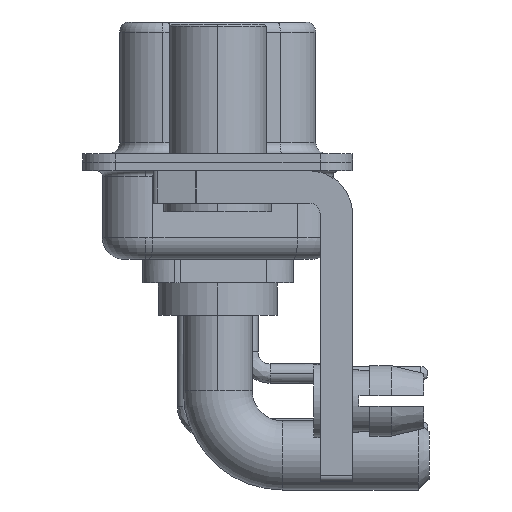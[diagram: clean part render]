
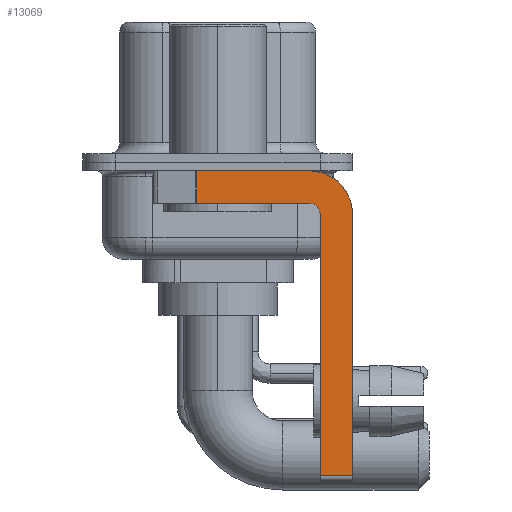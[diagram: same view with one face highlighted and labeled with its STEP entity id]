
A CAD part, left-side view. The second image highlights one B-rep face of the part: STEP entity #13069.
In plain terms, the highlighted planar face has unit normal (-1, 0, 0).
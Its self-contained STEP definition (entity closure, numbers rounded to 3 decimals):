
#56 = ORIENTED_EDGE ( 'NONE', *, *, #16880, .F. ) ;
#253 = AXIS2_PLACEMENT_3D ( 'NONE', #25060, #18763, #27129 ) ;
#539 = DIRECTION ( 'NONE',  ( 0., 0., 1. ) ) ;
#663 = ORIENTED_EDGE ( 'NONE', *, *, #20393, .F. ) ;
#1455 = DIRECTION ( 'NONE',  ( 0., -1., 0. ) ) ;
#1506 = CIRCLE ( 'NONE', #12465, 2. ) ;
#2091 = CARTESIAN_POINT ( 'NONE',  ( -2.9, -4.25, -2.4 ) ) ;
#2707 = VECTOR ( 'NONE', #539, 1000. ) ;
#2998 = VERTEX_POINT ( 'NONE', #23717 ) ;
#3106 = CARTESIAN_POINT ( 'NONE',  ( -2.9, 0.978, -0.4 ) ) ;
#3359 = FACE_OUTER_BOUND ( 'NONE', #25714, .T. ) ;
#3771 = DIRECTION ( 'NONE',  ( 0., 0., -1. ) ) ;
#4015 = DIRECTION ( 'NONE',  ( 1., 0., 0. ) ) ;
#4507 = VERTEX_POINT ( 'NONE', #8786 ) ;
#5295 = CARTESIAN_POINT ( 'NONE',  ( -2.9, 0.978, -1.9 ) ) ;
#5368 = EDGE_CURVE ( 'NONE', #7218, #7149, #9666, .T. ) ;
#5975 = CARTESIAN_POINT ( 'NONE',  ( -2.9, -4.25, -2.4 ) ) ;
#6104 = VECTOR ( 'NONE', #6245, 1000. ) ;
#6245 = DIRECTION ( 'NONE',  ( 0., 0., -1. ) ) ;
#6252 = VECTOR ( 'NONE', #26511, 1000. ) ;
#7069 = CARTESIAN_POINT ( 'NONE',  ( -2.9, -6.25, -14.55 ) ) ;
#7149 = VERTEX_POINT ( 'NONE', #7069 ) ;
#7218 = VERTEX_POINT ( 'NONE', #11446 ) ;
#8028 = CARTESIAN_POINT ( 'NONE',  ( -2.9, 3., -0.4 ) ) ;
#8734 = VERTEX_POINT ( 'NONE', #13606 ) ;
#8786 = CARTESIAN_POINT ( 'NONE',  ( -2.9, -4.25, -0.4 ) ) ;
#9634 = EDGE_CURVE ( 'NONE', #8734, #26486, #11653, .T. ) ;
#9666 = LINE ( 'NONE', #18153, #6252 ) ;
#10043 = ORIENTED_EDGE ( 'NONE', *, *, #9634, .F. ) ;
#10490 = CARTESIAN_POINT ( 'NONE',  ( -2.9, 0.978, -1.9 ) ) ;
#10621 = ORIENTED_EDGE ( 'NONE', *, *, #14471, .T. ) ;
#10810 = DIRECTION ( 'NONE',  ( 0., 0., -1. ) ) ;
#11446 = CARTESIAN_POINT ( 'NONE',  ( -2.9, -4.75, -14.55 ) ) ;
#11539 = VECTOR ( 'NONE', #10810, 1000. ) ;
#11653 = CIRCLE ( 'NONE', #253, 0.5 ) ;
#11730 = VECTOR ( 'NONE', #22242, 1000. ) ;
#12465 = AXIS2_PLACEMENT_3D ( 'NONE', #2091, #4015, #27053 ) ;
#12948 = LINE ( 'NONE', #10490, #6104 ) ;
#13045 = EDGE_CURVE ( 'NONE', #16100, #4507, #26399, .T. ) ;
#13069 = ADVANCED_FACE ( 'NONE', ( #3359 ), #18305, .F. ) ;
#13557 = ORIENTED_EDGE ( 'NONE', *, *, #21149, .F. ) ;
#13606 = CARTESIAN_POINT ( 'NONE',  ( -2.9, -4.75, -2.4 ) ) ;
#13901 = CARTESIAN_POINT ( 'NONE',  ( -2.9, -4.25, -1.9 ) ) ;
#14471 = EDGE_CURVE ( 'NONE', #16100, #23660, #12948, .T. ) ;
#14956 = ORIENTED_EDGE ( 'NONE', *, *, #23041, .F. ) ;
#15536 = ORIENTED_EDGE ( 'NONE', *, *, #5368, .T. ) ;
#15800 = CARTESIAN_POINT ( 'NONE',  ( -2.9, -4.25, -1.9 ) ) ;
#16100 = VERTEX_POINT ( 'NONE', #3106 ) ;
#16179 = AXIS2_PLACEMENT_3D ( 'NONE', #5975, #26677, #3771 ) ;
#16880 = EDGE_CURVE ( 'NONE', #7218, #8734, #25766, .T. ) ;
#17390 = CARTESIAN_POINT ( 'NONE',  ( -2.9, -6.25, -2.4 ) ) ;
#18153 = CARTESIAN_POINT ( 'NONE',  ( -2.9, -4.25, -14.55 ) ) ;
#18305 = PLANE ( 'NONE',  #16179 ) ;
#18763 = DIRECTION ( 'NONE',  ( -1., 0., 0. ) ) ;
#18925 = LINE ( 'NONE', #17390, #11539 ) ;
#20041 = ORIENTED_EDGE ( 'NONE', *, *, #13045, .F. ) ;
#20393 = EDGE_CURVE ( 'NONE', #2998, #7149, #18925, .T. ) ;
#21149 = EDGE_CURVE ( 'NONE', #4507, #2998, #1506, .T. ) ;
#21654 = CARTESIAN_POINT ( 'NONE',  ( -2.9, -4.75, -14.8 ) ) ;
#22242 = DIRECTION ( 'NONE',  ( 0., 1., 0. ) ) ;
#23041 = EDGE_CURVE ( 'NONE', #26486, #23660, #26648, .T. ) ;
#23660 = VERTEX_POINT ( 'NONE', #5295 ) ;
#23717 = CARTESIAN_POINT ( 'NONE',  ( -2.9, -6.25, -2.4 ) ) ;
#25060 = CARTESIAN_POINT ( 'NONE',  ( -2.9, -4.25, -2.4 ) ) ;
#25346 = VECTOR ( 'NONE', #1455, 1000. ) ;
#25714 = EDGE_LOOP ( 'NONE', ( #20041, #10621, #14956, #10043, #56, #15536, #663, #13557 ) ) ;
#25766 = LINE ( 'NONE', #21654, #2707 ) ;
#26399 = LINE ( 'NONE', #8028, #25346 ) ;
#26486 = VERTEX_POINT ( 'NONE', #15800 ) ;
#26511 = DIRECTION ( 'NONE',  ( 0., -1., 0. ) ) ;
#26648 = LINE ( 'NONE', #13901, #11730 ) ;
#26677 = DIRECTION ( 'NONE',  ( 1., 0., 0. ) ) ;
#27053 = DIRECTION ( 'NONE',  ( 0., 0., -1. ) ) ;
#27129 = DIRECTION ( 'NONE',  ( 0., 0., 1. ) ) ;
